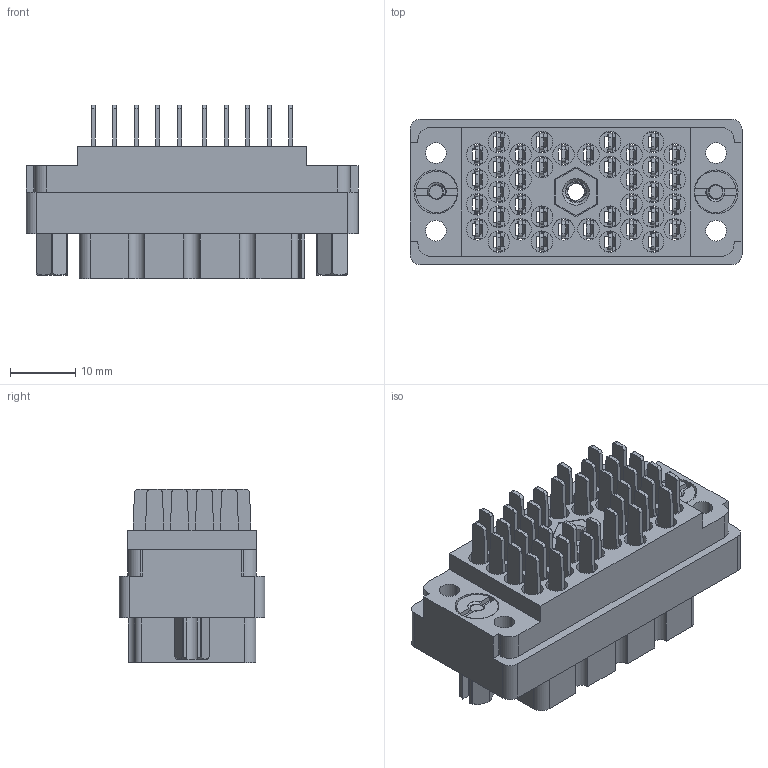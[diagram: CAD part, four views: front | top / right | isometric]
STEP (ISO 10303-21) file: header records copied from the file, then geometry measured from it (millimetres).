
FILE_DESCRIPTION (( 'STEP AP203' ), '1' );
FILE_NAME ('516-038-501-602.STEP', '2020-09-08T15:33:27', ( '' ), ( '' ), 'SwSTEP 2.0', 'SolidWorks 2020', '' );
FILE_SCHEMA (( 'CONFIG_CONTROL_DESIGN' ));
Length unit declared in the file: inch
Products named in the file (7): 516-292-001_501 Contact; 516-221-038-102_039; 516-038-501-602; 516-252-035-100_516-252-035-100; 516-221-038-102_038; 516-252-021-102_038; 516 Part Receptacle_038
Assembly tree (45 placements, depth 2):
  516-038-501-602
    516 Part Receptacle_038
    516-292-001_501 Contact  x39
    516-252-021-102_038  x2
    516-221-038-102_038
    516-252-035-100_516-252-035-100
    516-221-038-102_039
Bounding box: 50.8 x 22.25 x 26.49 mm (x, y, z)
Volume: 12765.5 mm3; surface area: 23133.5 mm2
Topology: 45 solids, 45 shells, 3945 faces, 11400 edges, 7560 vertices
Faces by surface type: plane 2294, cylinder 1339, bspline 268, cone 44
Entity records: 47447 total; most frequent: CARTESIAN_POINT 14165, ORIENTED_EDGE 6804, DIRECTION 6421, EDGE_CURVE 3402, VECTOR 2271, LINE 2271, VERTEX_POINT 2256, AXIS2_PLACEMENT_3D 2075
